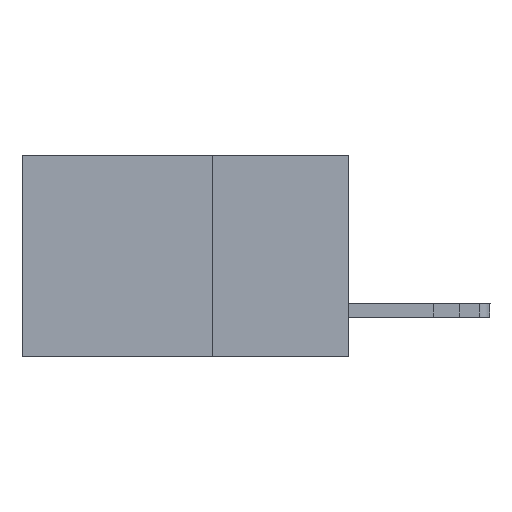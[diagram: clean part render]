
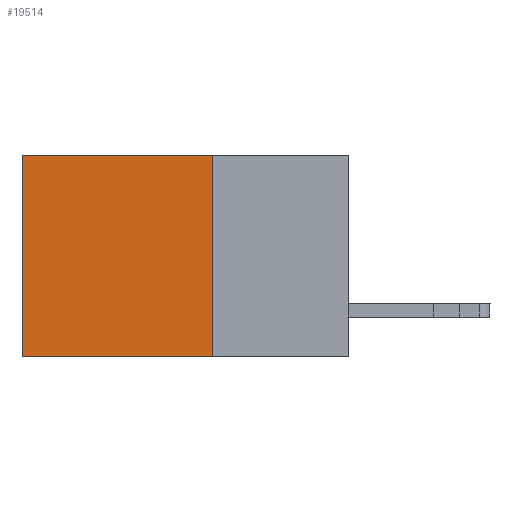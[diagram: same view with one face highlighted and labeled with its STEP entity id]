
A CAD part, left-side view. The second image highlights one B-rep face of the part: STEP entity #19514.
In plain terms, the highlighted planar face has unit normal (-1, 0, 0).
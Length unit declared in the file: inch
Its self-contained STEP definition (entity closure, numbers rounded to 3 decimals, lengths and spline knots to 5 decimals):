
#52 = VERTEX_POINT ( 'NONE', #4770 ) ;
#166 = DIRECTION ( 'NONE',  ( 0., 1., 0. ) ) ;
#683 = DIRECTION ( 'NONE',  ( 0., 0., -1. ) ) ;
#2580 = CARTESIAN_POINT ( 'NONE',  ( 0.298, 0.6, 0. ) ) ;
#4342 = FACE_OUTER_BOUND ( 'NONE', #18283, .T. ) ;
#4748 = ORIENTED_EDGE ( 'NONE', *, *, #5306, .F. ) ;
#4770 = CARTESIAN_POINT ( 'NONE',  ( 0.298, 0.25, -0.37 ) ) ;
#5306 = EDGE_CURVE ( 'NONE', #52, #24123, #5607, .T. ) ;
#5607 = LINE ( 'NONE', #18452, #17636 ) ;
#6871 = CARTESIAN_POINT ( 'NONE',  ( 0.298, 0.6, -0.37 ) ) ;
#8365 = DIRECTION ( 'NONE',  ( 1., 0., 0. ) ) ;
#8683 = DIRECTION ( 'NONE',  ( 0., 0., -1. ) ) ;
#10224 = CARTESIAN_POINT ( 'NONE',  ( 0.298, 0.25, 0. ) ) ;
#10878 = LINE ( 'NONE', #22007, #23229 ) ;
#12213 = VERTEX_POINT ( 'NONE', #10224 ) ;
#14006 = LINE ( 'NONE', #2580, #18718 ) ;
#14121 = ORIENTED_EDGE ( 'NONE', *, *, #20893, .F. ) ;
#14396 = ORIENTED_EDGE ( 'NONE', *, *, #22191, .T. ) ;
#14714 = LINE ( 'NONE', #22754, #20363 ) ;
#16349 = CARTESIAN_POINT ( 'NONE',  ( 0.298, 0.6, 0. ) ) ;
#16752 = PLANE ( 'NONE',  #19828 ) ;
#17636 = VECTOR ( 'NONE', #166, 39.37008 ) ;
#18283 = EDGE_LOOP ( 'NONE', ( #14396, #4748, #14121, #20013 ) ) ;
#18423 = CARTESIAN_POINT ( 'NONE',  ( 0.298, 0.25, 0. ) ) ;
#18452 = CARTESIAN_POINT ( 'NONE',  ( 0.298, 0.25, -0.37 ) ) ;
#18718 = VECTOR ( 'NONE', #683, 39.37008 ) ;
#19514 = ADVANCED_FACE ( 'NONE', ( #4342 ), #16752, .F. ) ;
#19828 = AXIS2_PLACEMENT_3D ( 'NONE', #18423, #8365, #22683 ) ;
#20013 = ORIENTED_EDGE ( 'NONE', *, *, #21212, .T. ) ;
#20363 = VECTOR ( 'NONE', #8683, 39.37008 ) ;
#20893 = EDGE_CURVE ( 'NONE', #12213, #52, #14714, .T. ) ;
#21212 = EDGE_CURVE ( 'NONE', #12213, #21444, #10878, .T. ) ;
#21444 = VERTEX_POINT ( 'NONE', #16349 ) ;
#22007 = CARTESIAN_POINT ( 'NONE',  ( 0.298, 0.25, 0. ) ) ;
#22191 = EDGE_CURVE ( 'NONE', #21444, #24123, #14006, .T. ) ;
#22683 = DIRECTION ( 'NONE',  ( 0., 0., -1. ) ) ;
#22754 = CARTESIAN_POINT ( 'NONE',  ( 0.298, 0.25, 0. ) ) ;
#23229 = VECTOR ( 'NONE', #23801, 39.37008 ) ;
#23801 = DIRECTION ( 'NONE',  ( 0., 1., 0. ) ) ;
#24123 = VERTEX_POINT ( 'NONE', #6871 ) ;
